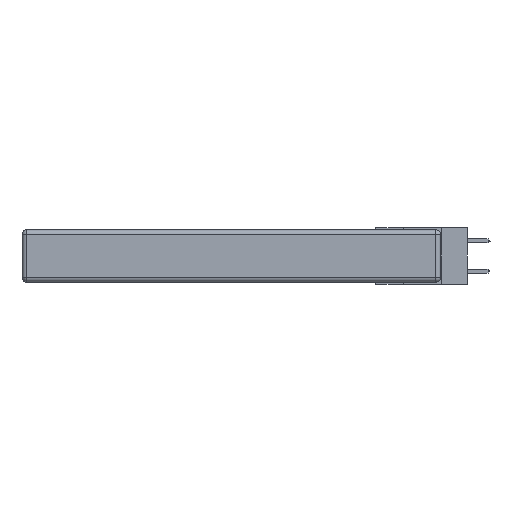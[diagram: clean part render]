
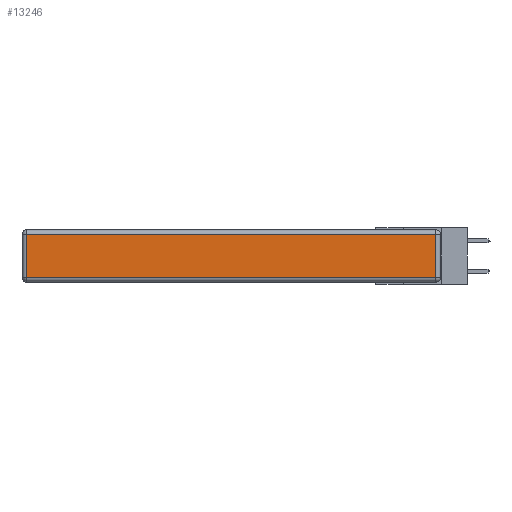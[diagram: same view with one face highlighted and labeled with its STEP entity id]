
A CAD part, left-side view. The second image highlights one B-rep face of the part: STEP entity #13246.
In plain terms, the highlighted planar face has unit normal (-1, 0, 0).
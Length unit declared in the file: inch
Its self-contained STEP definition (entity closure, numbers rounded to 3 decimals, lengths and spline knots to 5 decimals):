
#13 = VERTEX_POINT ( 'NONE', #8704 ) ;
#1089 = VERTEX_POINT ( 'NONE', #2606 ) ;
#1483 = ORIENTED_EDGE ( 'NONE', *, *, #9481, .T. ) ;
#1723 = ORIENTED_EDGE ( 'NONE', *, *, #7560, .T. ) ;
#2131 = CARTESIAN_POINT ( 'NONE',  ( 0., 2.72, -0.313 ) ) ;
#2446 = EDGE_LOOP ( 'NONE', ( #7316, #1483, #1723, #10219 ) ) ;
#2606 = CARTESIAN_POINT ( 'NONE',  ( 0., 0.03, -0.313 ) ) ;
#2675 = AXIS2_PLACEMENT_3D ( 'NONE', #15564, #8122, #15620 ) ;
#2681 = CARTESIAN_POINT ( 'NONE',  ( 0., 2.75, -0.03 ) ) ;
#3190 = VECTOR ( 'NONE', #3290, 39.37008 ) ;
#3290 = DIRECTION ( 'NONE',  ( 0., 0., 1. ) ) ;
#5799 = EDGE_CURVE ( 'NONE', #13, #11130, #15132, .T. ) ;
#6781 = DIRECTION ( 'NONE',  ( 0., 0., -1. ) ) ;
#7316 = ORIENTED_EDGE ( 'NONE', *, *, #12295, .T. ) ;
#7560 = EDGE_CURVE ( 'NONE', #12472, #13, #9420, .T. ) ;
#8122 = DIRECTION ( 'NONE',  ( -1., 0., 0. ) ) ;
#8358 = LINE ( 'NONE', #8906, #13598 ) ;
#8704 = CARTESIAN_POINT ( 'NONE',  ( 0., 2.72, -0.03 ) ) ;
#8906 = CARTESIAN_POINT ( 'NONE',  ( 0., 0., -0.313 ) ) ;
#9420 = LINE ( 'NONE', #2681, #9788 ) ;
#9481 = EDGE_CURVE ( 'NONE', #1089, #12472, #9748, .T. ) ;
#9748 = LINE ( 'NONE', #14342, #3190 ) ;
#9788 = VECTOR ( 'NONE', #15116, 39.37008 ) ;
#10219 = ORIENTED_EDGE ( 'NONE', *, *, #5799, .T. ) ;
#11130 = VERTEX_POINT ( 'NONE', #2131 ) ;
#11823 = FACE_OUTER_BOUND ( 'NONE', #2446, .T. ) ;
#11832 = CARTESIAN_POINT ( 'NONE',  ( 0., 0.03, -0.03 ) ) ;
#11981 = CARTESIAN_POINT ( 'NONE',  ( 0., 2.72, -0.343 ) ) ;
#12295 = EDGE_CURVE ( 'NONE', #11130, #1089, #8358, .T. ) ;
#12472 = VERTEX_POINT ( 'NONE', #11832 ) ;
#13246 = ADVANCED_FACE ( 'NONE', ( #11823 ), #14343, .T. ) ;
#13598 = VECTOR ( 'NONE', #13893, 39.37008 ) ;
#13893 = DIRECTION ( 'NONE',  ( 0., -1., 0. ) ) ;
#14342 = CARTESIAN_POINT ( 'NONE',  ( 0., 0.03, -0.343 ) ) ;
#14343 = PLANE ( 'NONE',  #2675 ) ;
#14948 = VECTOR ( 'NONE', #6781, 39.37008 ) ;
#15116 = DIRECTION ( 'NONE',  ( 0., 1., 0. ) ) ;
#15132 = LINE ( 'NONE', #11981, #14948 ) ;
#15564 = CARTESIAN_POINT ( 'NONE',  ( 0., 0., -0.343 ) ) ;
#15620 = DIRECTION ( 'NONE',  ( 0., 0., 1. ) ) ;
